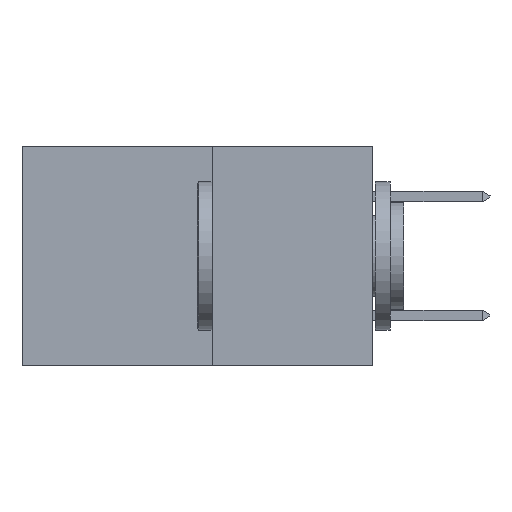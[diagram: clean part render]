
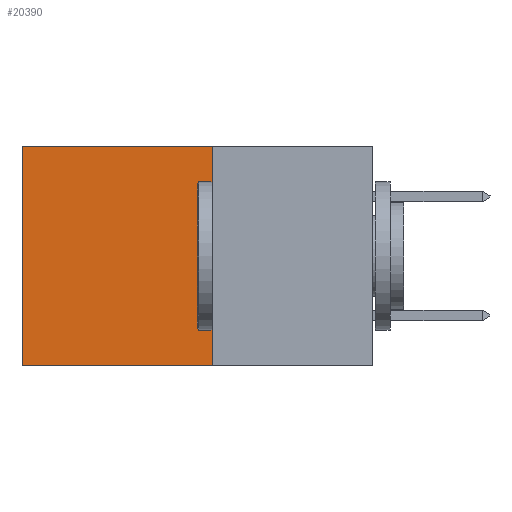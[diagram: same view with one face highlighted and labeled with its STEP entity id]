
A CAD part, left-side view. The second image highlights one B-rep face of the part: STEP entity #20390.
In plain terms, the highlighted planar face has unit normal (-1, 0, 0).
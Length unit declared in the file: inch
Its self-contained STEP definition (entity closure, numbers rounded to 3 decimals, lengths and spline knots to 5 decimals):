
#2114 = CARTESIAN_POINT ( 'NONE',  ( 0.277, 0.59, 0. ) ) ;
#2395 = CARTESIAN_POINT ( 'NONE',  ( 0.277, 0.27, -0.37 ) ) ;
#4124 = VECTOR ( 'NONE', #23469, 39.37008 ) ;
#5658 = VERTEX_POINT ( 'NONE', #5747 ) ;
#5747 = CARTESIAN_POINT ( 'NONE',  ( 0.277, 0.27, 0. ) ) ;
#5754 = ORIENTED_EDGE ( 'NONE', *, *, #16753, .T. ) ;
#6330 = DIRECTION ( 'NONE',  ( 0., 0., -1. ) ) ;
#6986 = PLANE ( 'NONE',  #7981 ) ;
#7576 = FACE_OUTER_BOUND ( 'NONE', #9991, .T. ) ;
#7883 = LINE ( 'NONE', #2395, #17273 ) ;
#7973 = CARTESIAN_POINT ( 'NONE',  ( 0.277, 0.27, -0.37 ) ) ;
#7981 = AXIS2_PLACEMENT_3D ( 'NONE', #20013, #10806, #23608 ) ;
#8904 = VECTOR ( 'NONE', #6330, 39.37008 ) ;
#9991 = EDGE_LOOP ( 'NONE', ( #5754, #10785, #17499, #18628 ) ) ;
#10785 = ORIENTED_EDGE ( 'NONE', *, *, #20108, .F. ) ;
#10806 = DIRECTION ( 'NONE',  ( 1., 0., 0. ) ) ;
#12056 = DIRECTION ( 'NONE',  ( 0., 0., -1. ) ) ;
#12536 = CARTESIAN_POINT ( 'NONE',  ( 0.277, 0.27, 0. ) ) ;
#13421 = EDGE_CURVE ( 'NONE', #5658, #16679, #20158, .T. ) ;
#13915 = LINE ( 'NONE', #15693, #8904 ) ;
#15347 = LINE ( 'NONE', #12536, #4124 ) ;
#15693 = CARTESIAN_POINT ( 'NONE',  ( 0.277, 0.59, -0.37 ) ) ;
#15857 = VERTEX_POINT ( 'NONE', #22487 ) ;
#15878 = VECTOR ( 'NONE', #12056, 39.37008 ) ;
#16679 = VERTEX_POINT ( 'NONE', #7973 ) ;
#16753 = EDGE_CURVE ( 'NONE', #20737, #15857, #13915, .T. ) ;
#17273 = VECTOR ( 'NONE', #21144, 39.37008 ) ;
#17499 = ORIENTED_EDGE ( 'NONE', *, *, #13421, .F. ) ;
#18274 = EDGE_CURVE ( 'NONE', #5658, #20737, #15347, .T. ) ;
#18628 = ORIENTED_EDGE ( 'NONE', *, *, #18274, .T. ) ;
#20013 = CARTESIAN_POINT ( 'NONE',  ( 0.277, 0.27, -0.37 ) ) ;
#20108 = EDGE_CURVE ( 'NONE', #16679, #15857, #7883, .T. ) ;
#20158 = LINE ( 'NONE', #22993, #15878 ) ;
#20390 = ADVANCED_FACE ( 'NONE', ( #7576 ), #6986, .F. ) ;
#20737 = VERTEX_POINT ( 'NONE', #2114 ) ;
#21144 = DIRECTION ( 'NONE',  ( 0., 1., 0. ) ) ;
#22487 = CARTESIAN_POINT ( 'NONE',  ( 0.277, 0.59, -0.37 ) ) ;
#22993 = CARTESIAN_POINT ( 'NONE',  ( 0.277, 0.27, -0.37 ) ) ;
#23469 = DIRECTION ( 'NONE',  ( 0., 1., 0. ) ) ;
#23608 = DIRECTION ( 'NONE',  ( 0., 0., -1. ) ) ;
